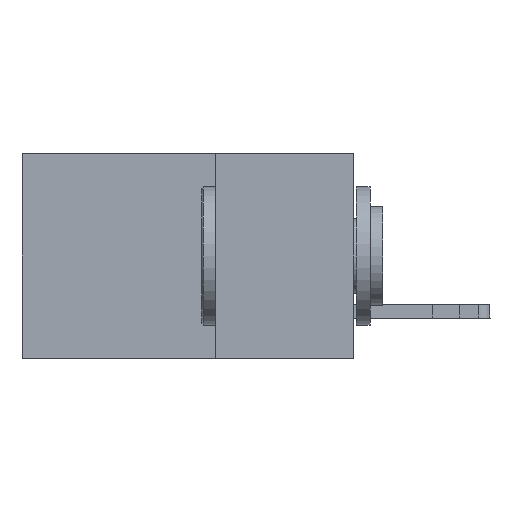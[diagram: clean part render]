
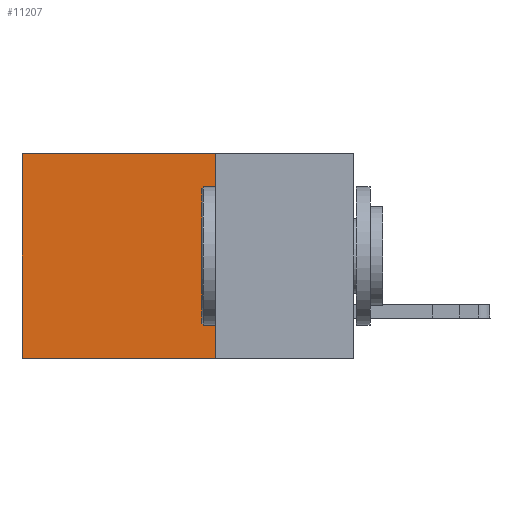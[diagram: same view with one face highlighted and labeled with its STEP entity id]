
A CAD part, left-side view. The second image highlights one B-rep face of the part: STEP entity #11207.
In plain terms, the highlighted planar face has unit normal (-1, 0, 0).
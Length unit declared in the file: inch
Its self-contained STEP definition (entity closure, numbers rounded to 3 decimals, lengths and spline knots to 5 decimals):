
#449 = ORIENTED_EDGE ( 'NONE', *, *, #13664, .F. ) ;
#1138 = VERTEX_POINT ( 'NONE', #31665 ) ;
#3408 = CARTESIAN_POINT ( 'NONE',  ( 0.2875, 0.6, 0. ) ) ;
#6599 = LINE ( 'NONE', #29961, #32697 ) ;
#6713 = CARTESIAN_POINT ( 'NONE',  ( 0.2875, 0.25, -0.37 ) ) ;
#8551 = VECTOR ( 'NONE', #18474, 39.37008 ) ;
#8834 = LINE ( 'NONE', #27743, #17525 ) ;
#10164 = ORIENTED_EDGE ( 'NONE', *, *, #24630, .T. ) ;
#10886 = CARTESIAN_POINT ( 'NONE',  ( 0.2875, 0.6, 0. ) ) ;
#11092 = VECTOR ( 'NONE', #18168, 39.37008 ) ;
#11207 = ADVANCED_FACE ( 'NONE', ( #17580 ), #17905, .F. ) ;
#11674 = DIRECTION ( 'NONE',  ( 0., 0., -1. ) ) ;
#13089 = LINE ( 'NONE', #31028, #11092 ) ;
#13664 = EDGE_CURVE ( 'NONE', #14046, #24333, #8834, .T. ) ;
#14046 = VERTEX_POINT ( 'NONE', #6713 ) ;
#15749 = EDGE_CURVE ( 'NONE', #21809, #24333, #26602, .T. ) ;
#17525 = VECTOR ( 'NONE', #19946, 39.37008 ) ;
#17580 = FACE_OUTER_BOUND ( 'NONE', #23263, .T. ) ;
#17905 = PLANE ( 'NONE',  #20102 ) ;
#18168 = DIRECTION ( 'NONE',  ( 0., 1., 0. ) ) ;
#18474 = DIRECTION ( 'NONE',  ( 0., 0., -1. ) ) ;
#19221 = CARTESIAN_POINT ( 'NONE',  ( 0.2875, 0.6, -0.37 ) ) ;
#19656 = ORIENTED_EDGE ( 'NONE', *, *, #15749, .T. ) ;
#19938 = DIRECTION ( 'NONE',  ( 1., 0., 0. ) ) ;
#19946 = DIRECTION ( 'NONE',  ( 0., 1., 0. ) ) ;
#20102 = AXIS2_PLACEMENT_3D ( 'NONE', #25521, #19938, #20113 ) ;
#20113 = DIRECTION ( 'NONE',  ( 0., 0., -1. ) ) ;
#21809 = VERTEX_POINT ( 'NONE', #10886 ) ;
#22284 = ORIENTED_EDGE ( 'NONE', *, *, #24096, .F. ) ;
#23263 = EDGE_LOOP ( 'NONE', ( #19656, #449, #22284, #10164 ) ) ;
#24096 = EDGE_CURVE ( 'NONE', #1138, #14046, #6599, .T. ) ;
#24333 = VERTEX_POINT ( 'NONE', #19221 ) ;
#24630 = EDGE_CURVE ( 'NONE', #1138, #21809, #13089, .T. ) ;
#25521 = CARTESIAN_POINT ( 'NONE',  ( 0.2875, 0.25, 0. ) ) ;
#26602 = LINE ( 'NONE', #3408, #8551 ) ;
#27743 = CARTESIAN_POINT ( 'NONE',  ( 0.2875, 0.25, -0.37 ) ) ;
#29961 = CARTESIAN_POINT ( 'NONE',  ( 0.2875, 0.25, 0. ) ) ;
#31028 = CARTESIAN_POINT ( 'NONE',  ( 0.2875, 0.25, 0. ) ) ;
#31665 = CARTESIAN_POINT ( 'NONE',  ( 0.2875, 0.25, 0. ) ) ;
#32697 = VECTOR ( 'NONE', #11674, 39.37008 ) ;
